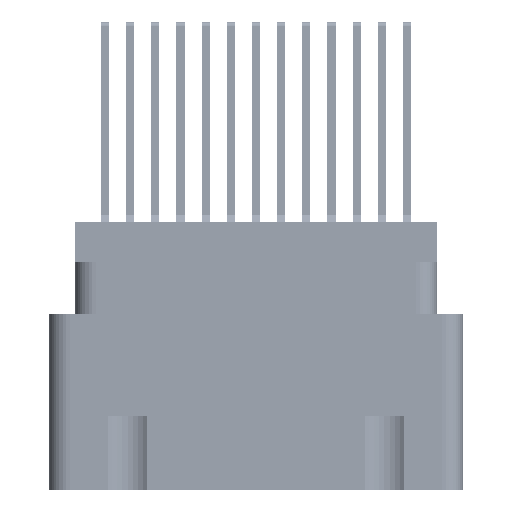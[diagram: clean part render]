
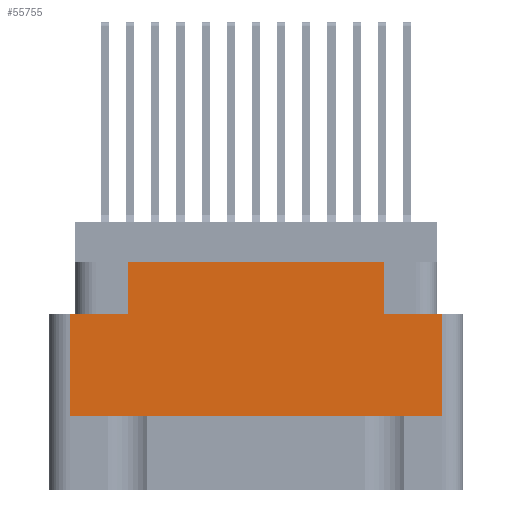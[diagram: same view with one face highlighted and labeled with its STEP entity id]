
A CAD part, left-side view. The second image highlights one B-rep face of the part: STEP entity #55755.
In plain terms, the highlighted planar face has unit normal (-1, 0, 0).
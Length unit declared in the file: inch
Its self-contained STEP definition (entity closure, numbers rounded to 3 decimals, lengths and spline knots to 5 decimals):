
#435 = VERTEX_POINT ( 'NONE', #36575 ) ;
#538 = DIRECTION ( 'NONE',  ( 0., 0., 1. ) ) ;
#1538 = CARTESIAN_POINT ( 'NONE',  ( -1.359, -0.3825, -0.117 ) ) ;
#2338 = DIRECTION ( 'NONE',  ( 0., 0., 1. ) ) ;
#2376 = ORIENTED_EDGE ( 'NONE', *, *, #54920, .T. ) ;
#2633 = EDGE_CURVE ( 'NONE', #25453, #33027, #63318, .T. ) ;
#3102 = VECTOR ( 'NONE', #538, 39.37008 ) ;
#3667 = DIRECTION ( 'NONE',  ( 0., 0., 1. ) ) ;
#3934 = VECTOR ( 'NONE', #3667, 39.37008 ) ;
#4165 = EDGE_CURVE ( 'NONE', #53662, #23301, #30341, .T. ) ;
#6642 = CARTESIAN_POINT ( 'NONE',  ( -1.359, 0.555, -0.578 ) ) ;
#9652 = VERTEX_POINT ( 'NONE', #6642 ) ;
#12549 = FACE_OUTER_BOUND ( 'NONE', #14249, .T. ) ;
#13920 = VECTOR ( 'NONE', #59293, 39.37008 ) ;
#14249 = EDGE_LOOP ( 'NONE', ( #67954, #37427, #46124, #2376, #17716, #50934, #58672, #60804 ) ) ;
#14910 = EDGE_CURVE ( 'NONE', #33027, #53662, #22049, .T. ) ;
#15179 = CARTESIAN_POINT ( 'NONE',  ( -1.359, -0.617, -0.798 ) ) ;
#15969 = CARTESIAN_POINT ( 'NONE',  ( -1.359, -0.3825, -0.274 ) ) ;
#16435 = EDGE_CURVE ( 'NONE', #25453, #9652, #17642, .T. ) ;
#17204 = AXIS2_PLACEMENT_3D ( 'NONE', #15179, #25962, #51852 ) ;
#17642 = LINE ( 'NONE', #20922, #44777 ) ;
#17716 = ORIENTED_EDGE ( 'NONE', *, *, #38350, .F. ) ;
#19425 = VERTEX_POINT ( 'NONE', #40773 ) ;
#20007 = PLANE ( 'NONE',  #17204 ) ;
#20922 = CARTESIAN_POINT ( 'NONE',  ( -1.359, 0.555, -0.798 ) ) ;
#22049 = LINE ( 'NONE', #34487, #3934 ) ;
#22402 = CARTESIAN_POINT ( 'NONE',  ( -1.359, 0.555, -0.274 ) ) ;
#23301 = VERTEX_POINT ( 'NONE', #1538 ) ;
#25453 = VERTEX_POINT ( 'NONE', #22402 ) ;
#25962 = DIRECTION ( 'NONE',  ( -1., 0., 0. ) ) ;
#27258 = CARTESIAN_POINT ( 'NONE',  ( -1.359, 0., -0.578 ) ) ;
#28973 = VECTOR ( 'NONE', #41421, 39.37008 ) ;
#30341 = LINE ( 'NONE', #38694, #31991 ) ;
#31991 = VECTOR ( 'NONE', #45310, 39.37008 ) ;
#33027 = VERTEX_POINT ( 'NONE', #57209 ) ;
#33885 = LINE ( 'NONE', #44423, #42094 ) ;
#34487 = CARTESIAN_POINT ( 'NONE',  ( -1.359, 0.3825, -0.274 ) ) ;
#36217 = VERTEX_POINT ( 'NONE', #63418 ) ;
#36575 = CARTESIAN_POINT ( 'NONE',  ( -1.359, -0.3825, -0.274 ) ) ;
#36980 = DIRECTION ( 'NONE',  ( 0., 0., -1. ) ) ;
#37427 = ORIENTED_EDGE ( 'NONE', *, *, #16435, .T. ) ;
#38350 = EDGE_CURVE ( 'NONE', #435, #36217, #38597, .T. ) ;
#38597 = LINE ( 'NONE', #45633, #13920 ) ;
#38694 = CARTESIAN_POINT ( 'NONE',  ( -1.359, 0.617, -0.117 ) ) ;
#40570 = VECTOR ( 'NONE', #58818, 39.37008 ) ;
#40773 = CARTESIAN_POINT ( 'NONE',  ( -1.359, -0.555, -0.578 ) ) ;
#41421 = DIRECTION ( 'NONE',  ( 0., -1., 0. ) ) ;
#42094 = VECTOR ( 'NONE', #2338, 39.37008 ) ;
#44423 = CARTESIAN_POINT ( 'NONE',  ( -1.359, -0.555, -0.798 ) ) ;
#44777 = VECTOR ( 'NONE', #36980, 39.37008 ) ;
#45310 = DIRECTION ( 'NONE',  ( 0., -1., 0. ) ) ;
#45633 = CARTESIAN_POINT ( 'NONE',  ( -1.359, 0., -0.274 ) ) ;
#46124 = ORIENTED_EDGE ( 'NONE', *, *, #46505, .T. ) ;
#46505 = EDGE_CURVE ( 'NONE', #9652, #19425, #52821, .T. ) ;
#46567 = CARTESIAN_POINT ( 'NONE',  ( -1.359, 0., -0.274 ) ) ;
#50934 = ORIENTED_EDGE ( 'NONE', *, *, #52537, .T. ) ;
#51852 = DIRECTION ( 'NONE',  ( 0., 0., 1. ) ) ;
#52537 = EDGE_CURVE ( 'NONE', #435, #23301, #56449, .T. ) ;
#52821 = LINE ( 'NONE', #27258, #40570 ) ;
#53662 = VERTEX_POINT ( 'NONE', #63933 ) ;
#54920 = EDGE_CURVE ( 'NONE', #19425, #36217, #33885, .T. ) ;
#55755 = ADVANCED_FACE ( 'NONE', ( #12549 ), #20007, .T. ) ;
#56449 = LINE ( 'NONE', #15969, #3102 ) ;
#57209 = CARTESIAN_POINT ( 'NONE',  ( -1.359, 0.3825, -0.274 ) ) ;
#58672 = ORIENTED_EDGE ( 'NONE', *, *, #4165, .F. ) ;
#58818 = DIRECTION ( 'NONE',  ( 0., -1., 0. ) ) ;
#59293 = DIRECTION ( 'NONE',  ( 0., -1., 0. ) ) ;
#60804 = ORIENTED_EDGE ( 'NONE', *, *, #14910, .F. ) ;
#63318 = LINE ( 'NONE', #46567, #28973 ) ;
#63418 = CARTESIAN_POINT ( 'NONE',  ( -1.359, -0.555, -0.274 ) ) ;
#63933 = CARTESIAN_POINT ( 'NONE',  ( -1.359, 0.3825, -0.117 ) ) ;
#67954 = ORIENTED_EDGE ( 'NONE', *, *, #2633, .F. ) ;
